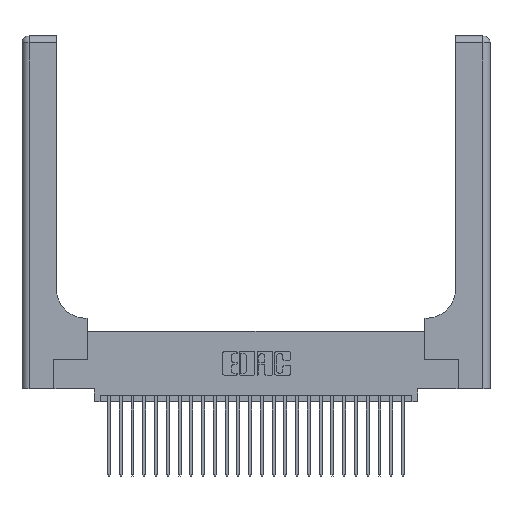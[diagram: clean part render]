
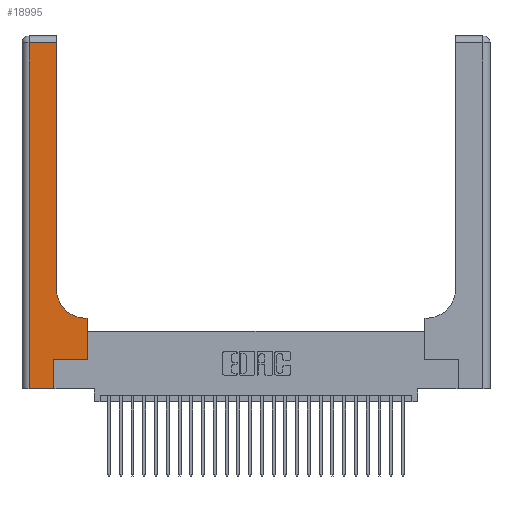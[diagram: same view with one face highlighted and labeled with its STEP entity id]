
A CAD part, top view. The second image highlights one B-rep face of the part: STEP entity #18995.
In plain terms, the highlighted planar face has unit normal (0, 0, 1).
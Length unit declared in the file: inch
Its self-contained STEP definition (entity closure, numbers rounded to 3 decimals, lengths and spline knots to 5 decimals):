
#235 = AXIS2_PLACEMENT_3D ( 'NONE', #10180, #25109, #12328 ) ;
#1044 = EDGE_CURVE ( 'NONE', #8558, #14106, #21419, .T. ) ;
#1427 = CARTESIAN_POINT ( 'NONE',  ( 0.06, 0., 0.37 ) ) ;
#1511 = CARTESIAN_POINT ( 'NONE',  ( 0.2915, 2.94, 0.37 ) ) ;
#1539 = DIRECTION ( 'NONE',  ( 0., -1., 0. ) ) ;
#2450 = EDGE_LOOP ( 'NONE', ( #7824, #10218, #4720, #23723, #7753, #21986, #11951, #18011, #19446 ) ) ;
#2599 = VERTEX_POINT ( 'NONE', #7889 ) ;
#3291 = DIRECTION ( 'NONE',  ( -1., 0., 0. ) ) ;
#3331 = VERTEX_POINT ( 'NONE', #3660 ) ;
#3611 = CARTESIAN_POINT ( 'NONE',  ( 0.2915, 3., 0.37 ) ) ;
#3660 = CARTESIAN_POINT ( 'NONE',  ( 0.269, 0., 0.37 ) ) ;
#3862 = VERTEX_POINT ( 'NONE', #1427 ) ;
#4057 = LINE ( 'NONE', #5242, #9917 ) ;
#4234 = VECTOR ( 'NONE', #6740, 39.37008 ) ;
#4720 = ORIENTED_EDGE ( 'NONE', *, *, #12935, .T. ) ;
#4729 = CARTESIAN_POINT ( 'NONE',  ( 0.2915, 0.85, 0.37 ) ) ;
#4773 = DIRECTION ( 'NONE',  ( -1., 0., 0. ) ) ;
#5234 = VERTEX_POINT ( 'NONE', #10279 ) ;
#5242 = CARTESIAN_POINT ( 'NONE',  ( 0.269, 0., 0.37 ) ) ;
#5293 = VECTOR ( 'NONE', #3291, 39.37008 ) ;
#5454 = LINE ( 'NONE', #26558, #16319 ) ;
#6372 = VECTOR ( 'NONE', #1539, 39.37008 ) ;
#6740 = DIRECTION ( 'NONE',  ( 0., 1., 0. ) ) ;
#7753 = ORIENTED_EDGE ( 'NONE', *, *, #13999, .T. ) ;
#7824 = ORIENTED_EDGE ( 'NONE', *, *, #9203, .T. ) ;
#7889 = CARTESIAN_POINT ( 'NONE',  ( 0.5585, 0.6, 0.37 ) ) ;
#7997 = PLANE ( 'NONE',  #235 ) ;
#8558 = VERTEX_POINT ( 'NONE', #1511 ) ;
#9093 = DIRECTION ( 'NONE',  ( 0., 0., -1. ) ) ;
#9203 = EDGE_CURVE ( 'NONE', #9526, #8558, #22692, .T. ) ;
#9526 = VERTEX_POINT ( 'NONE', #4729 ) ;
#9917 = VECTOR ( 'NONE', #20181, 39.37008 ) ;
#10095 = LINE ( 'NONE', #15338, #4234 ) ;
#10180 = CARTESIAN_POINT ( 'NONE',  ( 0., 3., 0.37 ) ) ;
#10218 = ORIENTED_EDGE ( 'NONE', *, *, #1044, .T. ) ;
#10279 = CARTESIAN_POINT ( 'NONE',  ( 0.5585, 0.25, 0.37 ) ) ;
#10632 = VECTOR ( 'NONE', #16718, 39.37008 ) ;
#11388 = AXIS2_PLACEMENT_3D ( 'NONE', #21942, #9093, #24049 ) ;
#11484 = LINE ( 'NONE', #14589, #6372 ) ;
#11951 = ORIENTED_EDGE ( 'NONE', *, *, #27880, .T. ) ;
#12128 = VECTOR ( 'NONE', #14258, 39.37008 ) ;
#12189 = CARTESIAN_POINT ( 'NONE',  ( 0.06, 2.94, 0.37 ) ) ;
#12328 = DIRECTION ( 'NONE',  ( -1., 0., 0. ) ) ;
#12935 = EDGE_CURVE ( 'NONE', #14106, #3862, #11484, .T. ) ;
#13452 = LINE ( 'NONE', #16457, #12128 ) ;
#13772 = DIRECTION ( 'NONE',  ( 1., 0., 0. ) ) ;
#13954 = EDGE_CURVE ( 'NONE', #16609, #5234, #5454, .T. ) ;
#13999 = EDGE_CURVE ( 'NONE', #3331, #16609, #4057, .T. ) ;
#14106 = VERTEX_POINT ( 'NONE', #12189 ) ;
#14258 = DIRECTION ( 'NONE',  ( 1., 0., 0. ) ) ;
#14589 = CARTESIAN_POINT ( 'NONE',  ( 0.06, 3., 0.37 ) ) ;
#14593 = EDGE_CURVE ( 'NONE', #14911, #9526, #25570, .T. ) ;
#14911 = VERTEX_POINT ( 'NONE', #20733 ) ;
#15338 = CARTESIAN_POINT ( 'NONE',  ( 0.5585, 0.25, 0.37 ) ) ;
#16314 = CARTESIAN_POINT ( 'NONE',  ( 0.2915, 0.6, 0.37 ) ) ;
#16319 = VECTOR ( 'NONE', #13772, 39.37008 ) ;
#16457 = CARTESIAN_POINT ( 'NONE',  ( 0., 0., 0.37 ) ) ;
#16609 = VERTEX_POINT ( 'NONE', #22221 ) ;
#16718 = DIRECTION ( 'NONE',  ( 0., 1., 0. ) ) ;
#16825 = LINE ( 'NONE', #16314, #5293 ) ;
#18011 = ORIENTED_EDGE ( 'NONE', *, *, #27598, .T. ) ;
#18995 = ADVANCED_FACE ( 'NONE', ( #27288 ), #7997, .F. ) ;
#19446 = ORIENTED_EDGE ( 'NONE', *, *, #14593, .T. ) ;
#19601 = EDGE_CURVE ( 'NONE', #3862, #3331, #13452, .T. ) ;
#20181 = DIRECTION ( 'NONE',  ( 0., 1., 0. ) ) ;
#20733 = CARTESIAN_POINT ( 'NONE',  ( 0.5415, 0.6, 0.37 ) ) ;
#21419 = LINE ( 'NONE', #26195, #25707 ) ;
#21942 = CARTESIAN_POINT ( 'NONE',  ( 0.5415, 0.85, 0.37 ) ) ;
#21986 = ORIENTED_EDGE ( 'NONE', *, *, #13954, .T. ) ;
#22221 = CARTESIAN_POINT ( 'NONE',  ( 0.269, 0.25, 0.37 ) ) ;
#22692 = LINE ( 'NONE', #3611, #10632 ) ;
#23723 = ORIENTED_EDGE ( 'NONE', *, *, #19601, .T. ) ;
#24049 = DIRECTION ( 'NONE',  ( 1., 0., 0. ) ) ;
#25109 = DIRECTION ( 'NONE',  ( 0., 0., -1. ) ) ;
#25570 = CIRCLE ( 'NONE', #11388, 0.25 ) ;
#25707 = VECTOR ( 'NONE', #4773, 39.37008 ) ;
#26195 = CARTESIAN_POINT ( 'NONE',  ( 0., 2.94, 0.37 ) ) ;
#26558 = CARTESIAN_POINT ( 'NONE',  ( 0.269, 0.25, 0.37 ) ) ;
#27288 = FACE_OUTER_BOUND ( 'NONE', #2450, .T. ) ;
#27598 = EDGE_CURVE ( 'NONE', #2599, #14911, #16825, .T. ) ;
#27880 = EDGE_CURVE ( 'NONE', #5234, #2599, #10095, .T. ) ;
